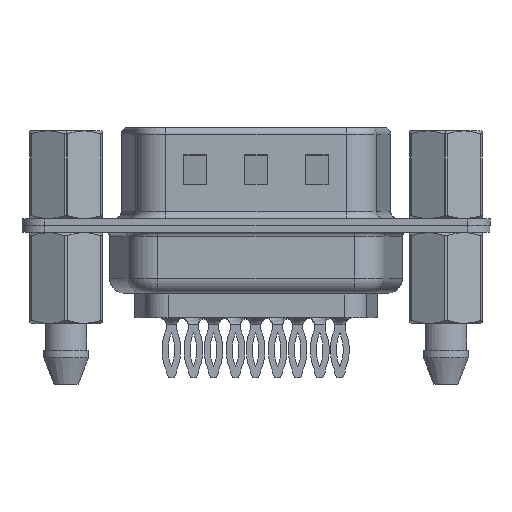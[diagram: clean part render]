
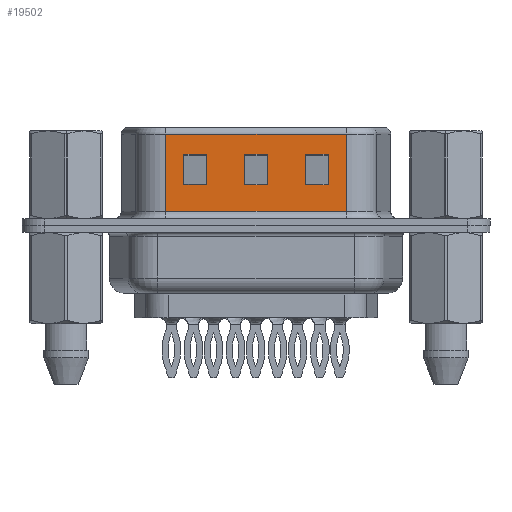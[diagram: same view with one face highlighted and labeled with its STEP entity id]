
A CAD part, front view. The second image highlights one B-rep face of the part: STEP entity #19502.
In plain terms, the highlighted planar face has unit normal (0, -1, 0).
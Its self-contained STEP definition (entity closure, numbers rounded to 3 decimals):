
#88 = ORIENTED_EDGE ( 'NONE', *, *, #20560, .T. ) ;
#371 = CARTESIAN_POINT ( 'NONE',  ( 18.445, -4.58, 6.02 ) ) ;
#571 = VECTOR ( 'NONE', #18561, 1000. ) ;
#589 = VERTEX_POINT ( 'NONE', #21854 ) ;
#898 = VERTEX_POINT ( 'NONE', #9168 ) ;
#953 = CARTESIAN_POINT ( 'NONE',  ( 22.445, -4.58, 4.705 ) ) ;
#1224 = EDGE_CURVE ( 'NONE', #18098, #6940, #22294, .T. ) ;
#1488 = DIRECTION ( 'NONE',  ( 0., 0., 1. ) ) ;
#1504 = LINE ( 'NONE', #953, #19471 ) ;
#2320 = CARTESIAN_POINT ( 'NONE',  ( 18.445, -4.58, 6.52 ) ) ;
#2370 = DIRECTION ( 'NONE',  ( 0., 0., -1. ) ) ;
#2554 = VECTOR ( 'NONE', #4457, 1000. ) ;
#2598 = CARTESIAN_POINT ( 'NONE',  ( 7.745, -4.58, 2.705 ) ) ;
#2899 = LINE ( 'NONE', #3250, #13674 ) ;
#2926 = CARTESIAN_POINT ( 'NONE',  ( 18.445, -4.58, 6.52 ) ) ;
#3098 = LINE ( 'NONE', #5052, #21546 ) ;
#3250 = CARTESIAN_POINT ( 'NONE',  ( 11.745, -4.58, 6.52 ) ) ;
#3278 = VECTOR ( 'NONE', #6146, 1000. ) ;
#3467 = DIRECTION ( 'NONE',  ( 1., 0., 0. ) ) ;
#3667 = LINE ( 'NONE', #12817, #9903 ) ;
#3759 = LINE ( 'NONE', #371, #21222 ) ;
#3992 = CARTESIAN_POINT ( 'NONE',  ( 6.545, -4.58, 0.95 ) ) ;
#4143 = ORIENTED_EDGE ( 'NONE', *, *, #22753, .T. ) ;
#4207 = EDGE_CURVE ( 'NONE', #11328, #6997, #1504, .T. ) ;
#4333 = CARTESIAN_POINT ( 'NONE',  ( 9.245, -4.58, 2.705 ) ) ;
#4457 = DIRECTION ( 'NONE',  ( -1., 0., 0. ) ) ;
#4459 = VECTOR ( 'NONE', #4878, 1000. ) ;
#4547 = CARTESIAN_POINT ( 'NONE',  ( 22.445, -4.58, 2.705 ) ) ;
#4614 = EDGE_CURVE ( 'NONE', #9481, #11328, #16349, .T. ) ;
#4639 = DIRECTION ( 'NONE',  ( 0., 0., -1. ) ) ;
#4659 = PLANE ( 'NONE',  #21834 ) ;
#4878 = DIRECTION ( 'NONE',  ( 0., 0., -1. ) ) ;
#5052 = CARTESIAN_POINT ( 'NONE',  ( 6.545, -4.58, 6.52 ) ) ;
#5434 = EDGE_CURVE ( 'NONE', #8059, #5490, #3667, .T. ) ;
#5490 = VERTEX_POINT ( 'NONE', #4333 ) ;
#5834 = ORIENTED_EDGE ( 'NONE', *, *, #18986, .T. ) ;
#5952 = VECTOR ( 'NONE', #9668, 1000. ) ;
#6115 = VERTEX_POINT ( 'NONE', #8100 ) ;
#6146 = DIRECTION ( 'NONE',  ( 0., 0., -1. ) ) ;
#6163 = VECTOR ( 'NONE', #4639, 1000. ) ;
#6382 = ORIENTED_EDGE ( 'NONE', *, *, #9322, .T. ) ;
#6433 = EDGE_LOOP ( 'NONE', ( #18908, #5834, #17074, #22854 ) ) ;
#6494 = LINE ( 'NONE', #17052, #6163 ) ;
#6608 = ORIENTED_EDGE ( 'NONE', *, *, #16179, .T. ) ;
#6917 = CARTESIAN_POINT ( 'NONE',  ( 18.445, -4.58, 2.705 ) ) ;
#6940 = VERTEX_POINT ( 'NONE', #10833 ) ;
#6968 = ORIENTED_EDGE ( 'NONE', *, *, #4614, .T. ) ;
#6997 = VERTEX_POINT ( 'NONE', #18459 ) ;
#7459 = DIRECTION ( 'NONE',  ( -1., 0., 0. ) ) ;
#8059 = VERTEX_POINT ( 'NONE', #20946 ) ;
#8100 = CARTESIAN_POINT ( 'NONE',  ( 11.745, -4.58, 4.705 ) ) ;
#8103 = EDGE_CURVE ( 'NONE', #6115, #14165, #8999, .T. ) ;
#8147 = FACE_BOUND ( 'NONE', #22770, .T. ) ;
#8270 = DIRECTION ( 'NONE',  ( 0., 1., 0. ) ) ;
#8765 = CARTESIAN_POINT ( 'NONE',  ( 18.445, -4.58, 4.705 ) ) ;
#8999 = LINE ( 'NONE', #8765, #19160 ) ;
#9153 = CARTESIAN_POINT ( 'NONE',  ( 15.745, -4.58, 2.705 ) ) ;
#9168 = CARTESIAN_POINT ( 'NONE',  ( 11.745, -4.58, 2.705 ) ) ;
#9287 = EDGE_CURVE ( 'NONE', #15452, #21135, #22042, .T. ) ;
#9303 = VECTOR ( 'NONE', #3467, 1000. ) ;
#9322 = EDGE_CURVE ( 'NONE', #898, #6115, #2899, .T. ) ;
#9481 = VERTEX_POINT ( 'NONE', #9153 ) ;
#9668 = DIRECTION ( 'NONE',  ( 0., 0., 1. ) ) ;
#9709 = ORIENTED_EDGE ( 'NONE', *, *, #4207, .T. ) ;
#9826 = ORIENTED_EDGE ( 'NONE', *, *, #12843, .T. ) ;
#9903 = VECTOR ( 'NONE', #2370, 1000. ) ;
#10002 = CARTESIAN_POINT ( 'NONE',  ( 15.745, -4.58, 4.705 ) ) ;
#10013 = DIRECTION ( 'NONE',  ( -1., 0., 0. ) ) ;
#10124 = LINE ( 'NONE', #13712, #4459 ) ;
#10443 = CARTESIAN_POINT ( 'NONE',  ( 18.445, -4.58, 0.95 ) ) ;
#10470 = DIRECTION ( 'NONE',  ( 1., 0., 0. ) ) ;
#10833 = CARTESIAN_POINT ( 'NONE',  ( 7.745, -4.58, 4.705 ) ) ;
#10842 = EDGE_LOOP ( 'NONE', ( #13857, #15509, #9826, #4143 ) ) ;
#10989 = CARTESIAN_POINT ( 'NONE',  ( 18.445, -4.58, 0.95 ) ) ;
#11243 = CARTESIAN_POINT ( 'NONE',  ( 14.445, -4.58, 4.705 ) ) ;
#11328 = VERTEX_POINT ( 'NONE', #10002 ) ;
#11592 = VERTEX_POINT ( 'NONE', #20659 ) ;
#11696 = ORIENTED_EDGE ( 'NONE', *, *, #13125, .T. ) ;
#11747 = LINE ( 'NONE', #4547, #19711 ) ;
#11858 = CARTESIAN_POINT ( 'NONE',  ( 7.745, -4.58, 6.52 ) ) ;
#11887 = EDGE_CURVE ( 'NONE', #11592, #898, #19104, .T. ) ;
#12585 = ORIENTED_EDGE ( 'NONE', *, *, #11887, .T. ) ;
#12817 = CARTESIAN_POINT ( 'NONE',  ( 9.245, -4.58, 6.52 ) ) ;
#12843 = EDGE_CURVE ( 'NONE', #16490, #22039, #3098, .T. ) ;
#13125 = EDGE_CURVE ( 'NONE', #589, #9481, #11747, .T. ) ;
#13383 = LINE ( 'NONE', #10443, #9303 ) ;
#13388 = FACE_BOUND ( 'NONE', #6433, .T. ) ;
#13674 = VECTOR ( 'NONE', #1488, 1000. ) ;
#13712 = CARTESIAN_POINT ( 'NONE',  ( 13.245, -4.58, 6.52 ) ) ;
#13857 = ORIENTED_EDGE ( 'NONE', *, *, #9287, .F. ) ;
#14165 = VERTEX_POINT ( 'NONE', #19862 ) ;
#15229 = FACE_OUTER_BOUND ( 'NONE', #10842, .T. ) ;
#15385 = EDGE_CURVE ( 'NONE', #15452, #16490, #3759, .T. ) ;
#15452 = VERTEX_POINT ( 'NONE', #21279 ) ;
#15509 = ORIENTED_EDGE ( 'NONE', *, *, #15385, .T. ) ;
#15848 = VECTOR ( 'NONE', #21891, 1000. ) ;
#16179 = EDGE_CURVE ( 'NONE', #6997, #589, #6494, .T. ) ;
#16284 = DIRECTION ( 'NONE',  ( 1., 0., 0. ) ) ;
#16349 = LINE ( 'NONE', #20180, #571 ) ;
#16490 = VERTEX_POINT ( 'NONE', #20149 ) ;
#17052 = CARTESIAN_POINT ( 'NONE',  ( 17.245, -4.58, 6.52 ) ) ;
#17074 = ORIENTED_EDGE ( 'NONE', *, *, #1224, .T. ) ;
#17076 = DIRECTION ( 'NONE',  ( 0., 0., 1. ) ) ;
#17754 = ORIENTED_EDGE ( 'NONE', *, *, #8103, .T. ) ;
#17804 = EDGE_CURVE ( 'NONE', #6940, #8059, #18529, .T. ) ;
#18098 = VERTEX_POINT ( 'NONE', #2598 ) ;
#18459 = CARTESIAN_POINT ( 'NONE',  ( 17.245, -4.58, 4.705 ) ) ;
#18529 = LINE ( 'NONE', #11243, #15848 ) ;
#18561 = DIRECTION ( 'NONE',  ( 0., 0., 1. ) ) ;
#18908 = ORIENTED_EDGE ( 'NONE', *, *, #5434, .T. ) ;
#18986 = EDGE_CURVE ( 'NONE', #5490, #18098, #20356, .T. ) ;
#19104 = LINE ( 'NONE', #6917, #21883 ) ;
#19160 = VECTOR ( 'NONE', #16284, 1000. ) ;
#19471 = VECTOR ( 'NONE', #10470, 1000. ) ;
#19502 = ADVANCED_FACE ( 'NONE', ( #13388, #20452, #8147, #15229 ), #4659, .F. ) ;
#19711 = VECTOR ( 'NONE', #10013, 1000. ) ;
#19862 = CARTESIAN_POINT ( 'NONE',  ( 13.245, -4.58, 4.705 ) ) ;
#20012 = CARTESIAN_POINT ( 'NONE',  ( 14.445, -4.58, 2.705 ) ) ;
#20149 = CARTESIAN_POINT ( 'NONE',  ( 6.545, -4.58, 6.02 ) ) ;
#20180 = CARTESIAN_POINT ( 'NONE',  ( 15.745, -4.58, 6.52 ) ) ;
#20356 = LINE ( 'NONE', #20012, #2554 ) ;
#20452 = FACE_BOUND ( 'NONE', #20835, .T. ) ;
#20516 = DIRECTION ( 'NONE',  ( -1., 0., 0. ) ) ;
#20560 = EDGE_CURVE ( 'NONE', #14165, #11592, #10124, .T. ) ;
#20659 = CARTESIAN_POINT ( 'NONE',  ( 13.245, -4.58, 2.705 ) ) ;
#20835 = EDGE_LOOP ( 'NONE', ( #6608, #11696, #6968, #9709 ) ) ;
#20946 = CARTESIAN_POINT ( 'NONE',  ( 9.245, -4.58, 4.705 ) ) ;
#21135 = VERTEX_POINT ( 'NONE', #10989 ) ;
#21222 = VECTOR ( 'NONE', #7459, 1000. ) ;
#21279 = CARTESIAN_POINT ( 'NONE',  ( 18.445, -4.58, 6.02 ) ) ;
#21546 = VECTOR ( 'NONE', #22452, 1000. ) ;
#21834 = AXIS2_PLACEMENT_3D ( 'NONE', #2926, #8270, #17076 ) ;
#21854 = CARTESIAN_POINT ( 'NONE',  ( 17.245, -4.58, 2.705 ) ) ;
#21883 = VECTOR ( 'NONE', #20516, 1000. ) ;
#21891 = DIRECTION ( 'NONE',  ( 1., 0., 0. ) ) ;
#22039 = VERTEX_POINT ( 'NONE', #3992 ) ;
#22042 = LINE ( 'NONE', #2320, #3278 ) ;
#22294 = LINE ( 'NONE', #11858, #5952 ) ;
#22452 = DIRECTION ( 'NONE',  ( 0., 0., -1. ) ) ;
#22753 = EDGE_CURVE ( 'NONE', #22039, #21135, #13383, .T. ) ;
#22770 = EDGE_LOOP ( 'NONE', ( #17754, #88, #12585, #6382 ) ) ;
#22854 = ORIENTED_EDGE ( 'NONE', *, *, #17804, .T. ) ;
